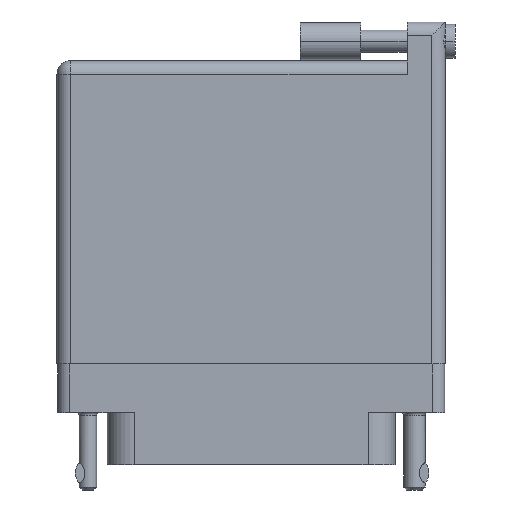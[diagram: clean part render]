
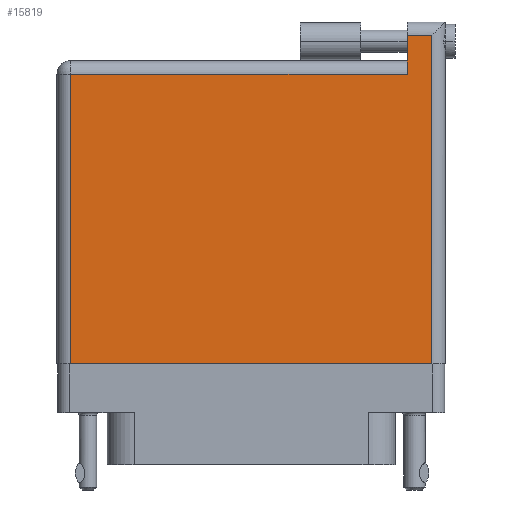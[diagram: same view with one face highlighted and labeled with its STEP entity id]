
A CAD part, front view. The second image highlights one B-rep face of the part: STEP entity #15819.
In plain terms, the highlighted face is planar.
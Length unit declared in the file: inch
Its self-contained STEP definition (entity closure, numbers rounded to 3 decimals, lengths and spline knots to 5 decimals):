
#382 = FACE_OUTER_BOUND ( 'NONE', #32184, .T. ) ;
#996 = ORIENTED_EDGE ( 'NONE', *, *, #8495, .T. ) ;
#1356 = CARTESIAN_POINT ( 'NONE',  ( -0.934, 1.396, 0.4495 ) ) ;
#1684 = CARTESIAN_POINT ( 'NONE',  ( -1.004, 1.596, 0.4495 ) ) ;
#4637 = DIRECTION ( 'NONE',  ( 0., 1., 0. ) ) ;
#4816 = DIRECTION ( 'NONE',  ( -1., 0., 0. ) ) ;
#7453 = CARTESIAN_POINT ( 'NONE',  ( 0.807, 1.666, 0.4495 ) ) ;
#8249 = DIRECTION ( 'NONE',  ( 0., 0., -1. ) ) ;
#8495 = EDGE_CURVE ( 'NONE', #29243, #48693, #15220, .T. ) ;
#8830 = CARTESIAN_POINT ( 'NONE',  ( 0.807, 1.596, 0.4495 ) ) ;
#11105 = DIRECTION ( 'NONE',  ( 0., -1., 0. ) ) ;
#12223 = CARTESIAN_POINT ( 'NONE',  ( 0.934, 1.666, 0.4495 ) ) ;
#13112 = CARTESIAN_POINT ( 'NONE',  ( -1.004, -0.1, 0.4495 ) ) ;
#13269 = LINE ( 'NONE', #28806, #26893 ) ;
#13345 = AXIS2_PLACEMENT_3D ( 'NONE', #24049, #8249, #4816 ) ;
#13778 = ORIENTED_EDGE ( 'NONE', *, *, #26885, .T. ) ;
#15178 = ORIENTED_EDGE ( 'NONE', *, *, #34404, .T. ) ;
#15220 = LINE ( 'NONE', #13112, #22387 ) ;
#15819 = ADVANCED_FACE ( 'NONE', ( #382 ), #46203, .F. ) ;
#16445 = VECTOR ( 'NONE', #47025, 39.37008 ) ;
#19230 = VERTEX_POINT ( 'NONE', #30286 ) ;
#20232 = EDGE_CURVE ( 'NONE', #34635, #29243, #21475, .T. ) ;
#21475 = LINE ( 'NONE', #40951, #33254 ) ;
#21925 = CARTESIAN_POINT ( 'NONE',  ( -0.934, -0.1, 0.4495 ) ) ;
#22048 = ORIENTED_EDGE ( 'NONE', *, *, #20232, .T. ) ;
#22057 = CARTESIAN_POINT ( 'NONE',  ( 0.934, -0.1, 0.4495 ) ) ;
#22387 = VECTOR ( 'NONE', #28206, 39.37008 ) ;
#24049 = CARTESIAN_POINT ( 'NONE',  ( -1.004, 1.466, 0.4495 ) ) ;
#24416 = VERTEX_POINT ( 'NONE', #32052 ) ;
#26026 = DIRECTION ( 'NONE',  ( 0., -1., 0. ) ) ;
#26531 = LINE ( 'NONE', #1684, #16445 ) ;
#26732 = EDGE_CURVE ( 'NONE', #48693, #19230, #34006, .T. ) ;
#26885 = EDGE_CURVE ( 'NONE', #24416, #34635, #13269, .T. ) ;
#26893 = VECTOR ( 'NONE', #44034, 39.37008 ) ;
#28206 = DIRECTION ( 'NONE',  ( 1., 0., 0. ) ) ;
#28798 = LINE ( 'NONE', #7453, #45361 ) ;
#28806 = CARTESIAN_POINT ( 'NONE',  ( -1.004, 1.396, 0.4495 ) ) ;
#29243 = VERTEX_POINT ( 'NONE', #21925 ) ;
#30286 = CARTESIAN_POINT ( 'NONE',  ( 0.934, 1.596, 0.4495 ) ) ;
#32052 = CARTESIAN_POINT ( 'NONE',  ( 0.807, 1.396, 0.4495 ) ) ;
#32184 = EDGE_LOOP ( 'NONE', ( #996, #33475, #37599, #15178, #13778, #22048 ) ) ;
#33254 = VECTOR ( 'NONE', #26026, 39.37008 ) ;
#33475 = ORIENTED_EDGE ( 'NONE', *, *, #26732, .T. ) ;
#33756 = EDGE_CURVE ( 'NONE', #19230, #43563, #26531, .T. ) ;
#34006 = LINE ( 'NONE', #12223, #41753 ) ;
#34404 = EDGE_CURVE ( 'NONE', #43563, #24416, #28798, .T. ) ;
#34635 = VERTEX_POINT ( 'NONE', #1356 ) ;
#37599 = ORIENTED_EDGE ( 'NONE', *, *, #33756, .T. ) ;
#40951 = CARTESIAN_POINT ( 'NONE',  ( -0.934, -0.1, 0.4495 ) ) ;
#41753 = VECTOR ( 'NONE', #4637, 39.37008 ) ;
#43563 = VERTEX_POINT ( 'NONE', #8830 ) ;
#44034 = DIRECTION ( 'NONE',  ( -1., 0., 0. ) ) ;
#45361 = VECTOR ( 'NONE', #11105, 39.37008 ) ;
#46203 = PLANE ( 'NONE',  #13345 ) ;
#47025 = DIRECTION ( 'NONE',  ( -1., 0., 0. ) ) ;
#48693 = VERTEX_POINT ( 'NONE', #22057 ) ;
